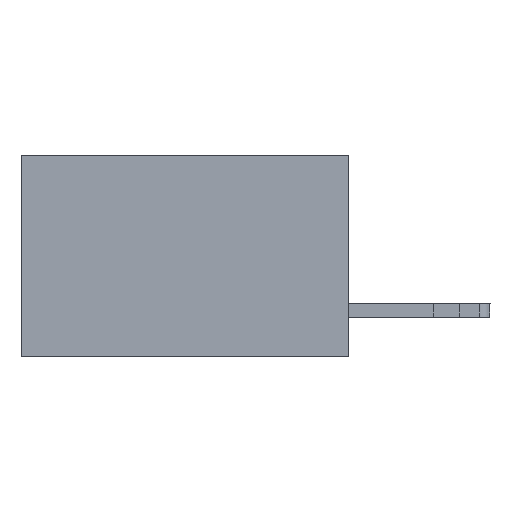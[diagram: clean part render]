
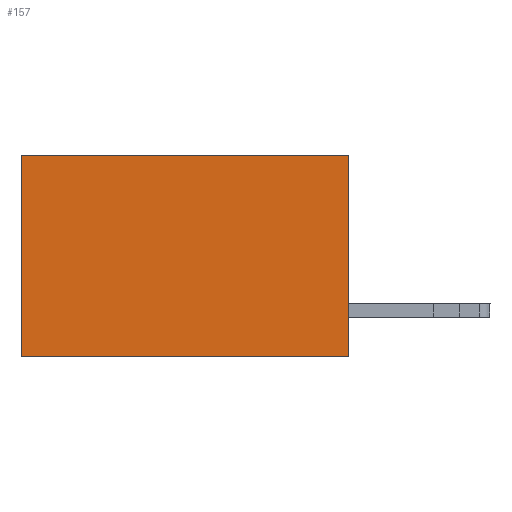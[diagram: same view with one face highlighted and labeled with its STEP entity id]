
A CAD part, left-side view. The second image highlights one B-rep face of the part: STEP entity #157.
In plain terms, the highlighted planar face has unit normal (-1, 0, 0).
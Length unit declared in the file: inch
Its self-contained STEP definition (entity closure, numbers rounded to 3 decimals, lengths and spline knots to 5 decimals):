
#88 = CARTESIAN_POINT ( 'NONE',  ( 0.2615, 0., 0. ) ) ;
#157 = ADVANCED_FACE ( 'NONE', ( #11339 ), #11224, .F. ) ;
#676 = VERTEX_POINT ( 'NONE', #14619 ) ;
#801 = LINE ( 'NONE', #6140, #12552 ) ;
#1206 = EDGE_LOOP ( 'NONE', ( #17223, #7196, #3296, #15414 ) ) ;
#1489 = VECTOR ( 'NONE', #5991, 39.37008 ) ;
#1572 = DIRECTION ( 'NONE',  ( 0., 1., 0. ) ) ;
#2544 = VERTEX_POINT ( 'NONE', #5481 ) ;
#3296 = ORIENTED_EDGE ( 'NONE', *, *, #9913, .F. ) ;
#3452 = CARTESIAN_POINT ( 'NONE',  ( 0.2615, 0.6, -0.37 ) ) ;
#3556 = LINE ( 'NONE', #15485, #7797 ) ;
#4035 = EDGE_CURVE ( 'NONE', #2544, #4906, #11562, .T. ) ;
#4401 = CARTESIAN_POINT ( 'NONE',  ( 0.2615, 0., -0.37 ) ) ;
#4906 = VERTEX_POINT ( 'NONE', #3452 ) ;
#5478 = DIRECTION ( 'NONE',  ( 0., 1., 0. ) ) ;
#5481 = CARTESIAN_POINT ( 'NONE',  ( 0.2615, 0.6, 0. ) ) ;
#5991 = DIRECTION ( 'NONE',  ( 0., 0., -1. ) ) ;
#6105 = VERTEX_POINT ( 'NONE', #14025 ) ;
#6140 = CARTESIAN_POINT ( 'NONE',  ( 0.2615, 0., -0.37 ) ) ;
#7196 = ORIENTED_EDGE ( 'NONE', *, *, #11762, .F. ) ;
#7797 = VECTOR ( 'NONE', #5478, 39.37008 ) ;
#9616 = DIRECTION ( 'NONE',  ( 1., 0., 0. ) ) ;
#9913 = EDGE_CURVE ( 'NONE', #676, #6105, #801, .T. ) ;
#11224 = PLANE ( 'NONE',  #13491 ) ;
#11339 = FACE_OUTER_BOUND ( 'NONE', #1206, .T. ) ;
#11562 = LINE ( 'NONE', #16563, #1489 ) ;
#11762 = EDGE_CURVE ( 'NONE', #6105, #4906, #3556, .T. ) ;
#12552 = VECTOR ( 'NONE', #14672, 39.37008 ) ;
#12647 = VECTOR ( 'NONE', #1572, 39.37008 ) ;
#13491 = AXIS2_PLACEMENT_3D ( 'NONE', #4401, #9616, #14994 ) ;
#14025 = CARTESIAN_POINT ( 'NONE',  ( 0.2615, 0., -0.37 ) ) ;
#14619 = CARTESIAN_POINT ( 'NONE',  ( 0.2615, 0., 0. ) ) ;
#14672 = DIRECTION ( 'NONE',  ( 0., 0., -1. ) ) ;
#14994 = DIRECTION ( 'NONE',  ( 0., 0., -1. ) ) ;
#15414 = ORIENTED_EDGE ( 'NONE', *, *, #15574, .T. ) ;
#15485 = CARTESIAN_POINT ( 'NONE',  ( 0.2615, 0., -0.37 ) ) ;
#15574 = EDGE_CURVE ( 'NONE', #676, #2544, #15781, .T. ) ;
#15781 = LINE ( 'NONE', #88, #12647 ) ;
#16563 = CARTESIAN_POINT ( 'NONE',  ( 0.2615, 0.6, -0.37 ) ) ;
#17223 = ORIENTED_EDGE ( 'NONE', *, *, #4035, .T. ) ;
